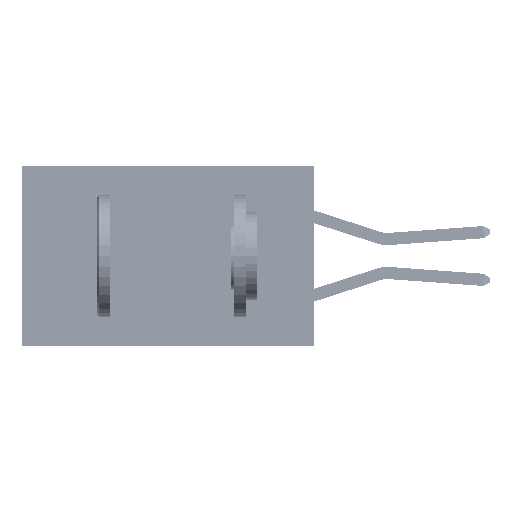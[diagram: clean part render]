
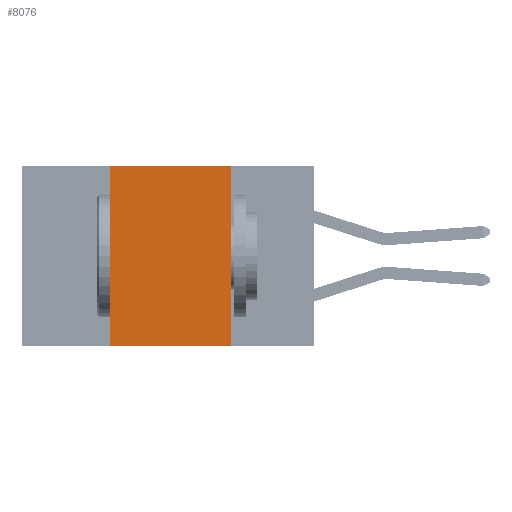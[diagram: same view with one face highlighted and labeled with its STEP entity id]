
A CAD part, left-side view. The second image highlights one B-rep face of the part: STEP entity #8076.
In plain terms, the highlighted planar face has unit normal (-1, 0, 0).
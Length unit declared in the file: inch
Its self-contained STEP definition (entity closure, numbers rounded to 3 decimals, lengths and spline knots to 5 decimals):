
#1222 = DIRECTION ( 'NONE',  ( 0., 0., -1. ) ) ;
#2350 = PLANE ( 'NONE',  #17873 ) ;
#3540 = CARTESIAN_POINT ( 'NONE',  ( 0., 0.42, 0. ) ) ;
#4344 = CARTESIAN_POINT ( 'NONE',  ( 0., 0.42, 0. ) ) ;
#4368 = LINE ( 'NONE', #4344, #4993 ) ;
#4993 = VECTOR ( 'NONE', #27690, 39.37008 ) ;
#6214 = CARTESIAN_POINT ( 'NONE',  ( 0., 0.6, 0. ) ) ;
#7752 = ORIENTED_EDGE ( 'NONE', *, *, #38554, .F. ) ;
#7789 = CARTESIAN_POINT ( 'NONE',  ( 0., 0.42, -0.37 ) ) ;
#8076 = ADVANCED_FACE ( 'NONE', ( #19141 ), #2350, .F. ) ;
#10894 = DIRECTION ( 'NONE',  ( 0., 0., -1. ) ) ;
#15552 = VERTEX_POINT ( 'NONE', #31668 ) ;
#16135 = DIRECTION ( 'NONE',  ( 0., -1., 0. ) ) ;
#17873 = AXIS2_PLACEMENT_3D ( 'NONE', #6214, #32903, #10894 ) ;
#18290 = ORIENTED_EDGE ( 'NONE', *, *, #32218, .F. ) ;
#19141 = FACE_OUTER_BOUND ( 'NONE', #47909, .T. ) ;
#19271 = VERTEX_POINT ( 'NONE', #42706 ) ;
#19693 = EDGE_CURVE ( 'NONE', #15552, #19271, #34283, .T. ) ;
#24121 = VECTOR ( 'NONE', #1222, 39.37008 ) ;
#27690 = DIRECTION ( 'NONE',  ( 0., 0., 1. ) ) ;
#27749 = CARTESIAN_POINT ( 'NONE',  ( 0., 0.17, 0. ) ) ;
#29769 = ORIENTED_EDGE ( 'NONE', *, *, #35327, .T. ) ;
#31637 = VERTEX_POINT ( 'NONE', #7789 ) ;
#31668 = CARTESIAN_POINT ( 'NONE',  ( 0., 0.17, 0. ) ) ;
#32218 = EDGE_CURVE ( 'NONE', #31637, #49255, #4368, .T. ) ;
#32775 = DIRECTION ( 'NONE',  ( 0., -1., 0. ) ) ;
#32903 = DIRECTION ( 'NONE',  ( 1., 0., 0. ) ) ;
#33326 = ORIENTED_EDGE ( 'NONE', *, *, #19693, .F. ) ;
#33833 = LINE ( 'NONE', #46693, #42810 ) ;
#34283 = LINE ( 'NONE', #27749, #24121 ) ;
#35327 = EDGE_CURVE ( 'NONE', #31637, #19271, #33833, .T. ) ;
#36580 = CARTESIAN_POINT ( 'NONE',  ( 0., 0.6, 0. ) ) ;
#37608 = VECTOR ( 'NONE', #32775, 39.37008 ) ;
#38554 = EDGE_CURVE ( 'NONE', #49255, #15552, #46588, .T. ) ;
#42706 = CARTESIAN_POINT ( 'NONE',  ( 0., 0.17, -0.37 ) ) ;
#42810 = VECTOR ( 'NONE', #16135, 39.37008 ) ;
#46588 = LINE ( 'NONE', #36580, #37608 ) ;
#46693 = CARTESIAN_POINT ( 'NONE',  ( 0., 0.6, -0.37 ) ) ;
#47909 = EDGE_LOOP ( 'NONE', ( #33326, #7752, #18290, #29769 ) ) ;
#49255 = VERTEX_POINT ( 'NONE', #3540 ) ;
